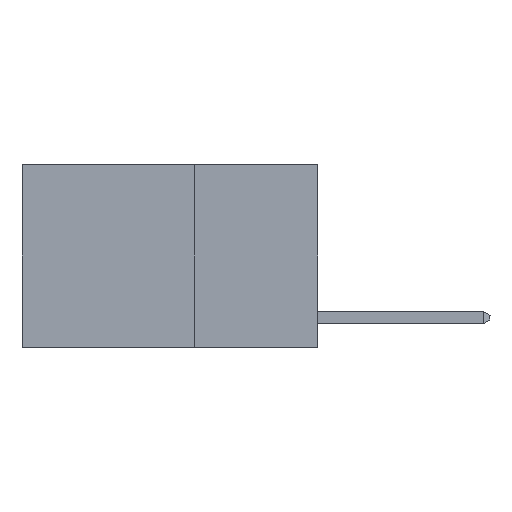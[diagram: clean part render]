
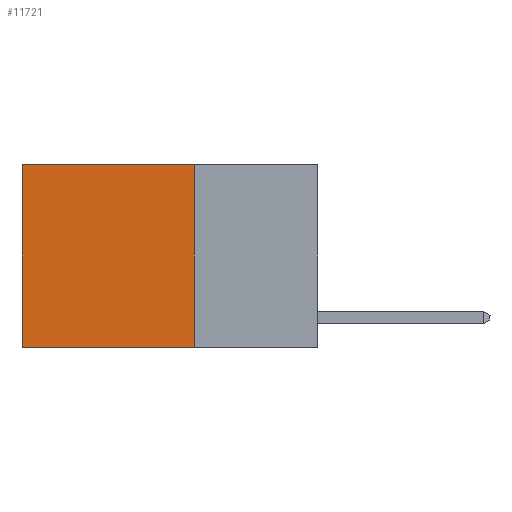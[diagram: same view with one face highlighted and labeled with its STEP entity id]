
A CAD part, left-side view. The second image highlights one B-rep face of the part: STEP entity #11721.
In plain terms, the highlighted planar face has unit normal (-1, 0, 0).
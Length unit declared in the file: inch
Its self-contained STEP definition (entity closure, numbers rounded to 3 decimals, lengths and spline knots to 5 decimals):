
#519 = CARTESIAN_POINT ( 'NONE',  ( 0.2625, 0.25, 0. ) ) ;
#848 = CARTESIAN_POINT ( 'NONE',  ( 0.2625, 0.6, 0. ) ) ;
#2138 = VERTEX_POINT ( 'NONE', #12991 ) ;
#2183 = FACE_OUTER_BOUND ( 'NONE', #19580, .T. ) ;
#4098 = DIRECTION ( 'NONE',  ( 0., 1., 0. ) ) ;
#4137 = DIRECTION ( 'NONE',  ( 0., 0., -1. ) ) ;
#5341 = DIRECTION ( 'NONE',  ( 0., 1., 0. ) ) ;
#6310 = CARTESIAN_POINT ( 'NONE',  ( 0.2625, 0.25, -0.37 ) ) ;
#7098 = ORIENTED_EDGE ( 'NONE', *, *, #20787, .F. ) ;
#7722 = CARTESIAN_POINT ( 'NONE',  ( 0.2625, 0.25, 0. ) ) ;
#8252 = EDGE_CURVE ( 'NONE', #10740, #17610, #16829, .T. ) ;
#9181 = EDGE_CURVE ( 'NONE', #9985, #17610, #16047, .T. ) ;
#9436 = CARTESIAN_POINT ( 'NONE',  ( 0.2625, 0.25, 0. ) ) ;
#9985 = VERTEX_POINT ( 'NONE', #848 ) ;
#10107 = AXIS2_PLACEMENT_3D ( 'NONE', #519, #13282, #17368 ) ;
#10258 = EDGE_CURVE ( 'NONE', #2138, #9985, #26378, .T. ) ;
#10540 = PLANE ( 'NONE',  #10107 ) ;
#10740 = VERTEX_POINT ( 'NONE', #21997 ) ;
#11387 = ORIENTED_EDGE ( 'NONE', *, *, #10258, .T. ) ;
#11721 = ADVANCED_FACE ( 'NONE', ( #2183 ), #10540, .F. ) ;
#12702 = VECTOR ( 'NONE', #5341, 39.37008 ) ;
#12991 = CARTESIAN_POINT ( 'NONE',  ( 0.2625, 0.25, 0. ) ) ;
#13282 = DIRECTION ( 'NONE',  ( 1., 0., 0. ) ) ;
#13869 = LINE ( 'NONE', #7722, #24266 ) ;
#14013 = CARTESIAN_POINT ( 'NONE',  ( 0.2625, 0.6, 0. ) ) ;
#16047 = LINE ( 'NONE', #14013, #26589 ) ;
#16829 = LINE ( 'NONE', #6310, #20513 ) ;
#17368 = DIRECTION ( 'NONE',  ( 0., 0., -1. ) ) ;
#17610 = VERTEX_POINT ( 'NONE', #19360 ) ;
#19360 = CARTESIAN_POINT ( 'NONE',  ( 0.2625, 0.6, -0.37 ) ) ;
#19580 = EDGE_LOOP ( 'NONE', ( #20492, #23062, #7098, #11387 ) ) ;
#20492 = ORIENTED_EDGE ( 'NONE', *, *, #9181, .T. ) ;
#20513 = VECTOR ( 'NONE', #4098, 39.37008 ) ;
#20787 = EDGE_CURVE ( 'NONE', #2138, #10740, #13869, .T. ) ;
#21997 = CARTESIAN_POINT ( 'NONE',  ( 0.2625, 0.25, -0.37 ) ) ;
#22245 = DIRECTION ( 'NONE',  ( 0., 0., -1. ) ) ;
#23062 = ORIENTED_EDGE ( 'NONE', *, *, #8252, .F. ) ;
#24266 = VECTOR ( 'NONE', #22245, 39.37008 ) ;
#26378 = LINE ( 'NONE', #9436, #12702 ) ;
#26589 = VECTOR ( 'NONE', #4137, 39.37008 ) ;
